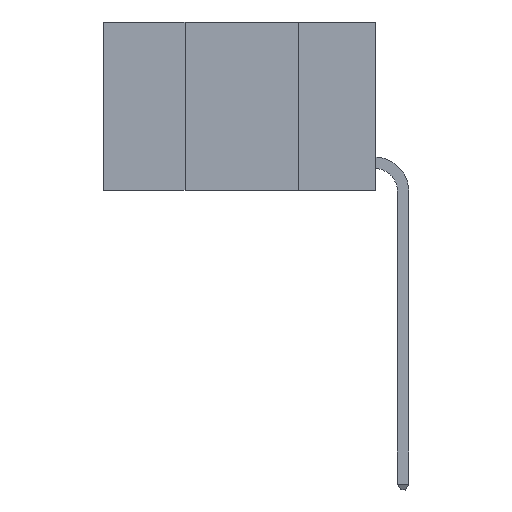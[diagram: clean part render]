
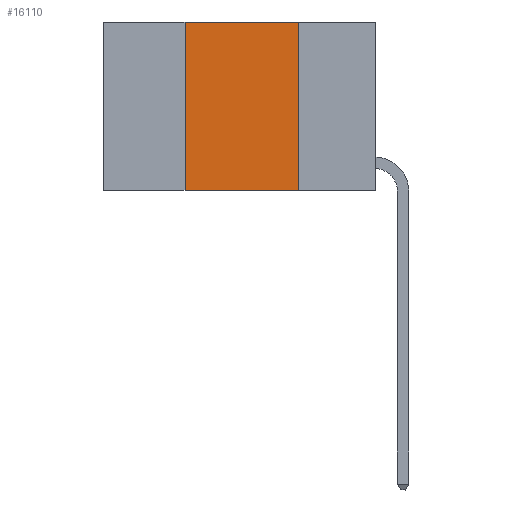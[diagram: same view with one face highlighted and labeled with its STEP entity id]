
A CAD part, left-side view. The second image highlights one B-rep face of the part: STEP entity #16110.
In plain terms, the highlighted planar face has unit normal (-1, 0, 0).
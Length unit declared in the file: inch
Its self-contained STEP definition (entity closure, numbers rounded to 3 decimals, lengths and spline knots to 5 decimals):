
#847 = CARTESIAN_POINT ( 'NONE',  ( 0., 0.42, 0. ) ) ;
#1008 = DIRECTION ( 'NONE',  ( 0., 0., 1. ) ) ;
#2011 = EDGE_CURVE ( 'NONE', #24791, #18109, #17528, .T. ) ;
#2299 = ORIENTED_EDGE ( 'NONE', *, *, #2011, .F. ) ;
#2543 = EDGE_LOOP ( 'NONE', ( #11087, #12810, #2299, #22535 ) ) ;
#3196 = VECTOR ( 'NONE', #20304, 39.37008 ) ;
#3995 = LINE ( 'NONE', #27361, #15462 ) ;
#5244 = CARTESIAN_POINT ( 'NONE',  ( 0., 0.17, 0. ) ) ;
#5855 = AXIS2_PLACEMENT_3D ( 'NONE', #19188, #10611, #25644 ) ;
#6073 = VECTOR ( 'NONE', #1008, 39.37008 ) ;
#7515 = CARTESIAN_POINT ( 'NONE',  ( 0., 0.42, 0. ) ) ;
#7652 = CARTESIAN_POINT ( 'NONE',  ( 0., 0.17, -0.37 ) ) ;
#10611 = DIRECTION ( 'NONE',  ( 1., 0., 0. ) ) ;
#11087 = ORIENTED_EDGE ( 'NONE', *, *, #21422, .F. ) ;
#11200 = VERTEX_POINT ( 'NONE', #26815 ) ;
#11369 = EDGE_CURVE ( 'NONE', #18109, #11200, #3995, .T. ) ;
#12810 = ORIENTED_EDGE ( 'NONE', *, *, #11369, .F. ) ;
#13998 = EDGE_CURVE ( 'NONE', #24791, #15217, #26409, .T. ) ;
#14021 = DIRECTION ( 'NONE',  ( 0., -1., 0. ) ) ;
#15217 = VERTEX_POINT ( 'NONE', #7652 ) ;
#15462 = VECTOR ( 'NONE', #20997, 39.37008 ) ;
#15686 = VECTOR ( 'NONE', #14021, 39.37008 ) ;
#15761 = CARTESIAN_POINT ( 'NONE',  ( 0., 0.42, -0.37 ) ) ;
#16110 = ADVANCED_FACE ( 'NONE', ( #18390 ), #17022, .F. ) ;
#17022 = PLANE ( 'NONE',  #5855 ) ;
#17528 = LINE ( 'NONE', #7515, #6073 ) ;
#18109 = VERTEX_POINT ( 'NONE', #847 ) ;
#18390 = FACE_OUTER_BOUND ( 'NONE', #2543, .T. ) ;
#19188 = CARTESIAN_POINT ( 'NONE',  ( 0., 0.6, 0. ) ) ;
#20304 = DIRECTION ( 'NONE',  ( 0., 0., -1. ) ) ;
#20997 = DIRECTION ( 'NONE',  ( 0., -1., 0. ) ) ;
#21422 = EDGE_CURVE ( 'NONE', #11200, #15217, #25456, .T. ) ;
#22535 = ORIENTED_EDGE ( 'NONE', *, *, #13998, .T. ) ;
#24791 = VERTEX_POINT ( 'NONE', #15761 ) ;
#25456 = LINE ( 'NONE', #5244, #3196 ) ;
#25644 = DIRECTION ( 'NONE',  ( 0., 0., -1. ) ) ;
#26409 = LINE ( 'NONE', #26859, #15686 ) ;
#26815 = CARTESIAN_POINT ( 'NONE',  ( 0., 0.17, 0. ) ) ;
#26859 = CARTESIAN_POINT ( 'NONE',  ( 0., 0.6, -0.37 ) ) ;
#27361 = CARTESIAN_POINT ( 'NONE',  ( 0., 0.6, 0. ) ) ;
